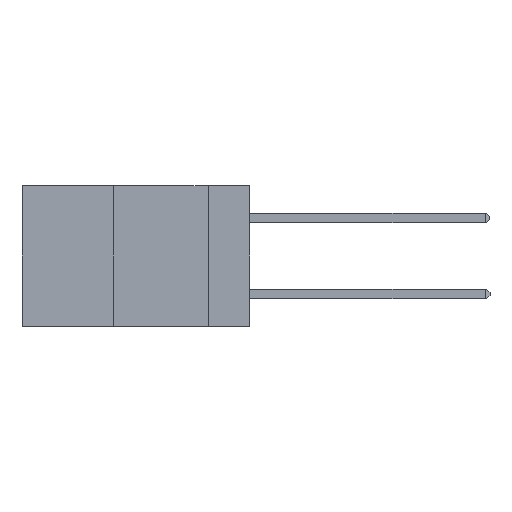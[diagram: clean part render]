
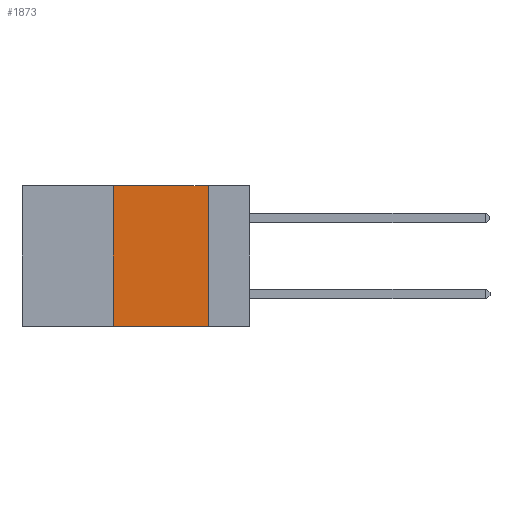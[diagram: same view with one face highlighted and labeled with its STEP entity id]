
A CAD part, left-side view. The second image highlights one B-rep face of the part: STEP entity #1873.
In plain terms, the highlighted planar face has unit normal (-1, 0, 0).
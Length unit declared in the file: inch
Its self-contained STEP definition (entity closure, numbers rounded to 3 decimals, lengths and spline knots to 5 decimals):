
#63 = VERTEX_POINT ( 'NONE', #13856 ) ;
#462 = VERTEX_POINT ( 'NONE', #11179 ) ;
#877 = CARTESIAN_POINT ( 'NONE',  ( 0., 0.6, 0. ) ) ;
#1873 = ADVANCED_FACE ( 'NONE', ( #14555 ), #7616, .F. ) ;
#2442 = ORIENTED_EDGE ( 'NONE', *, *, #12742, .F. ) ;
#2862 = AXIS2_PLACEMENT_3D ( 'NONE', #877, #15755, #14456 ) ;
#3306 = DIRECTION ( 'NONE',  ( 0., -1., 0. ) ) ;
#3467 = VECTOR ( 'NONE', #10747, 39.37008 ) ;
#3705 = LINE ( 'NONE', #12766, #10911 ) ;
#3816 = EDGE_CURVE ( 'NONE', #63, #16815, #15258, .T. ) ;
#4377 = EDGE_LOOP ( 'NONE', ( #2442, #14511, #16197, #7965 ) ) ;
#7024 = LINE ( 'NONE', #7991, #3467 ) ;
#7220 = DIRECTION ( 'NONE',  ( 0., 0., -1. ) ) ;
#7616 = PLANE ( 'NONE',  #2862 ) ;
#7965 = ORIENTED_EDGE ( 'NONE', *, *, #13294, .T. ) ;
#7991 = CARTESIAN_POINT ( 'NONE',  ( 0., 0.6, -0.37 ) ) ;
#8097 = VECTOR ( 'NONE', #14030, 39.37008 ) ;
#8192 = CARTESIAN_POINT ( 'NONE',  ( 0., 0.11, 0. ) ) ;
#9209 = LINE ( 'NONE', #15302, #11939 ) ;
#9731 = EDGE_CURVE ( 'NONE', #16815, #14439, #3705, .T. ) ;
#10747 = DIRECTION ( 'NONE',  ( 0., -1., 0. ) ) ;
#10911 = VECTOR ( 'NONE', #3306, 39.37008 ) ;
#11179 = CARTESIAN_POINT ( 'NONE',  ( 0., 0.11, -0.37 ) ) ;
#11939 = VECTOR ( 'NONE', #7220, 39.37008 ) ;
#12439 = CARTESIAN_POINT ( 'NONE',  ( 0., 0.36, 0. ) ) ;
#12742 = EDGE_CURVE ( 'NONE', #14439, #462, #9209, .T. ) ;
#12766 = CARTESIAN_POINT ( 'NONE',  ( 0., 0.6, 0. ) ) ;
#13294 = EDGE_CURVE ( 'NONE', #63, #462, #7024, .T. ) ;
#13856 = CARTESIAN_POINT ( 'NONE',  ( 0., 0.36, -0.37 ) ) ;
#14030 = DIRECTION ( 'NONE',  ( 0., 0., 1. ) ) ;
#14099 = CARTESIAN_POINT ( 'NONE',  ( 0., 0.36, 0. ) ) ;
#14439 = VERTEX_POINT ( 'NONE', #8192 ) ;
#14456 = DIRECTION ( 'NONE',  ( 0., 0., -1. ) ) ;
#14511 = ORIENTED_EDGE ( 'NONE', *, *, #9731, .F. ) ;
#14555 = FACE_OUTER_BOUND ( 'NONE', #4377, .T. ) ;
#15258 = LINE ( 'NONE', #14099, #8097 ) ;
#15302 = CARTESIAN_POINT ( 'NONE',  ( 0., 0.11, 0. ) ) ;
#15755 = DIRECTION ( 'NONE',  ( 1., 0., 0. ) ) ;
#16197 = ORIENTED_EDGE ( 'NONE', *, *, #3816, .F. ) ;
#16815 = VERTEX_POINT ( 'NONE', #12439 ) ;
